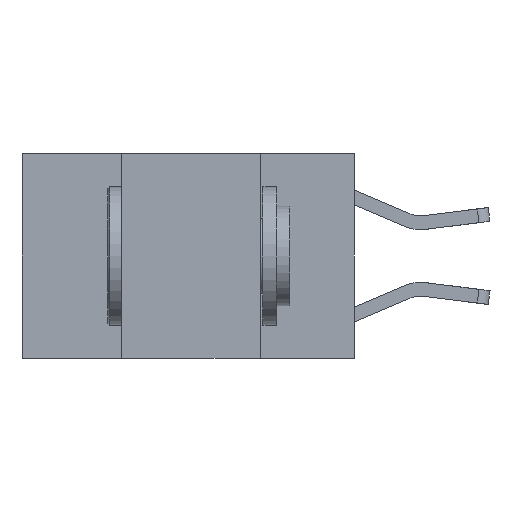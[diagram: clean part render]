
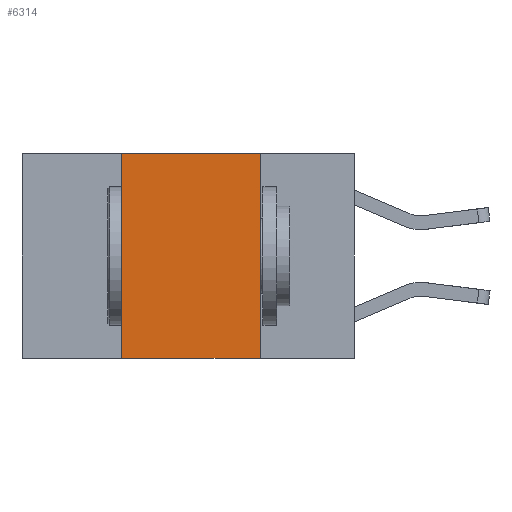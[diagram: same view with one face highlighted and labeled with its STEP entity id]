
A CAD part, left-side view. The second image highlights one B-rep face of the part: STEP entity #6314.
In plain terms, the highlighted planar face has unit normal (-1, 0, 0).
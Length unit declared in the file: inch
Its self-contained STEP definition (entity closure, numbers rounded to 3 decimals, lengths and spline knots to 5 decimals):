
#260 = VECTOR ( 'NONE', #1363, 39.37008 ) ;
#423 = ORIENTED_EDGE ( 'NONE', *, *, #3374, .F. ) ;
#474 = CARTESIAN_POINT ( 'NONE',  ( 0., 0.6, -0.37 ) ) ;
#514 = LINE ( 'NONE', #1678, #260 ) ;
#638 = CARTESIAN_POINT ( 'NONE',  ( 0., 0.6, 0. ) ) ;
#705 = AXIS2_PLACEMENT_3D ( 'NONE', #1461, #1327, #1293 ) ;
#954 = ORIENTED_EDGE ( 'NONE', *, *, #2156, .T. ) ;
#1010 = DIRECTION ( 'NONE',  ( 0., -1., 0. ) ) ;
#1293 = DIRECTION ( 'NONE',  ( 0., 0., -1. ) ) ;
#1327 = DIRECTION ( 'NONE',  ( 1., 0., 0. ) ) ;
#1363 = DIRECTION ( 'NONE',  ( 0., 0., -1. ) ) ;
#1420 = PLANE ( 'NONE',  #705 ) ;
#1461 = CARTESIAN_POINT ( 'NONE',  ( 0., 0.6, 0. ) ) ;
#1678 = CARTESIAN_POINT ( 'NONE',  ( 0., 0.17, 0. ) ) ;
#2156 = EDGE_CURVE ( 'NONE', #8833, #5069, #7118, .T. ) ;
#2171 = VERTEX_POINT ( 'NONE', #9615 ) ;
#2246 = LINE ( 'NONE', #638, #6020 ) ;
#2695 = EDGE_LOOP ( 'NONE', ( #6504, #423, #8702, #954 ) ) ;
#2980 = CARTESIAN_POINT ( 'NONE',  ( 0., 0.42, 0. ) ) ;
#3186 = EDGE_CURVE ( 'NONE', #8833, #5428, #3956, .T. ) ;
#3374 = EDGE_CURVE ( 'NONE', #5428, #2171, #2246, .T. ) ;
#3956 = LINE ( 'NONE', #5631, #9557 ) ;
#4462 = EDGE_CURVE ( 'NONE', #2171, #5069, #514, .T. ) ;
#4911 = DIRECTION ( 'NONE',  ( 0., 0., 1. ) ) ;
#5069 = VERTEX_POINT ( 'NONE', #6002 ) ;
#5428 = VERTEX_POINT ( 'NONE', #2980 ) ;
#5631 = CARTESIAN_POINT ( 'NONE',  ( 0., 0.42, 0. ) ) ;
#6002 = CARTESIAN_POINT ( 'NONE',  ( 0., 0.17, -0.37 ) ) ;
#6020 = VECTOR ( 'NONE', #1010, 39.37008 ) ;
#6314 = ADVANCED_FACE ( 'NONE', ( #6551 ), #1420, .F. ) ;
#6373 = DIRECTION ( 'NONE',  ( 0., -1., 0. ) ) ;
#6385 = VECTOR ( 'NONE', #6373, 39.37008 ) ;
#6504 = ORIENTED_EDGE ( 'NONE', *, *, #4462, .F. ) ;
#6551 = FACE_OUTER_BOUND ( 'NONE', #2695, .T. ) ;
#7118 = LINE ( 'NONE', #474, #6385 ) ;
#8702 = ORIENTED_EDGE ( 'NONE', *, *, #3186, .F. ) ;
#8833 = VERTEX_POINT ( 'NONE', #9105 ) ;
#9105 = CARTESIAN_POINT ( 'NONE',  ( 0., 0.42, -0.37 ) ) ;
#9557 = VECTOR ( 'NONE', #4911, 39.37008 ) ;
#9615 = CARTESIAN_POINT ( 'NONE',  ( 0., 0.17, 0. ) ) ;
